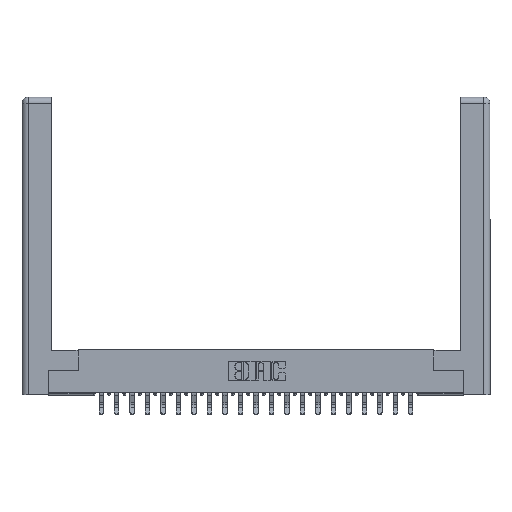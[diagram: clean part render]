
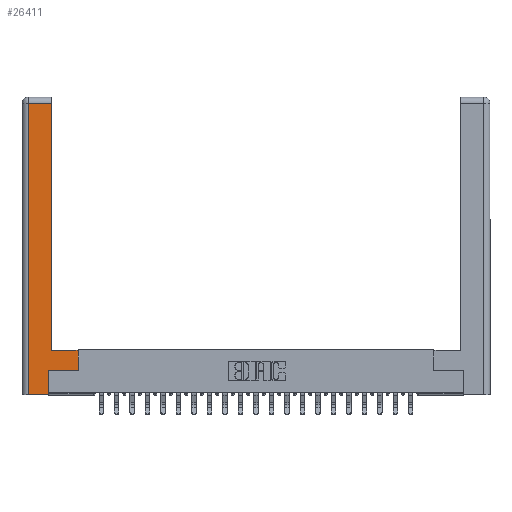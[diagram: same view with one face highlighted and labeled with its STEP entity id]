
A CAD part, top view. The second image highlights one B-rep face of the part: STEP entity #26411.
In plain terms, the highlighted planar face has unit normal (0, 0, 1).
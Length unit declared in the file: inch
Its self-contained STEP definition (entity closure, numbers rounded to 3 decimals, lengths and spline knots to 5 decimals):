
#15 = FACE_OUTER_BOUND ( 'NONE', #25318, .T. ) ;
#166 = ORIENTED_EDGE ( 'NONE', *, *, #12079, .T. ) ;
#227 = LINE ( 'NONE', #19545, #10065 ) ;
#1132 = CARTESIAN_POINT ( 'NONE',  ( 0.295, 0.45, 0. ) ) ;
#1381 = DIRECTION ( 'NONE',  ( 0., 1., 0. ) ) ;
#2128 = VERTEX_POINT ( 'NONE', #5772 ) ;
#2627 = ORIENTED_EDGE ( 'NONE', *, *, #8836, .T. ) ;
#3000 = EDGE_CURVE ( 'NONE', #23422, #21679, #227, .T. ) ;
#3068 = ORIENTED_EDGE ( 'NONE', *, *, #10850, .T. ) ;
#3162 = LINE ( 'NONE', #14942, #22546 ) ;
#4135 = EDGE_CURVE ( 'NONE', #21408, #21906, #3162, .T. ) ;
#4421 = DIRECTION ( 'NONE',  ( 0., -1., 0. ) ) ;
#4448 = ORIENTED_EDGE ( 'NONE', *, *, #3000, .T. ) ;
#5772 = CARTESIAN_POINT ( 'NONE',  ( 0.0615, 0., 0. ) ) ;
#6633 = DIRECTION ( 'NONE',  ( 0., 1., 0. ) ) ;
#8256 = CARTESIAN_POINT ( 'NONE',  ( 0.265, 0., 0. ) ) ;
#8334 = CARTESIAN_POINT ( 'NONE',  ( 0.565, 0.45, 0. ) ) ;
#8669 = DIRECTION ( 'NONE',  ( -1., 0., 0. ) ) ;
#8836 = EDGE_CURVE ( 'NONE', #23584, #11127, #10323, .T. ) ;
#9778 = VECTOR ( 'NONE', #18567, 39.37008 ) ;
#9855 = LINE ( 'NONE', #19994, #24811 ) ;
#10065 = VECTOR ( 'NONE', #6633, 39.37008 ) ;
#10323 = LINE ( 'NONE', #8334, #24931 ) ;
#10427 = DIRECTION ( 'NONE',  ( 0., 1., 0. ) ) ;
#10609 = DIRECTION ( 'NONE',  ( -1., 0., 0. ) ) ;
#10817 = AXIS2_PLACEMENT_3D ( 'NONE', #15261, #27907, #10609 ) ;
#10850 = EDGE_CURVE ( 'NONE', #2128, #23422, #20749, .T. ) ;
#11127 = VERTEX_POINT ( 'NONE', #22295 ) ;
#11364 = ORIENTED_EDGE ( 'NONE', *, *, #24656, .T. ) ;
#11489 = CARTESIAN_POINT ( 'NONE',  ( 0.295, 0.45, 0. ) ) ;
#11492 = LINE ( 'NONE', #20175, #9778 ) ;
#11603 = EDGE_CURVE ( 'NONE', #21906, #2128, #9855, .T. ) ;
#12079 = EDGE_CURVE ( 'NONE', #25902, #21408, #12204, .T. ) ;
#12204 = LINE ( 'NONE', #27332, #14255 ) ;
#12479 = ORIENTED_EDGE ( 'NONE', *, *, #16808, .T. ) ;
#12902 = DIRECTION ( 'NONE',  ( 1., 0., 0. ) ) ;
#13479 = CARTESIAN_POINT ( 'NONE',  ( 0.265, 0.245, 0. ) ) ;
#14255 = VECTOR ( 'NONE', #1381, 39.37008 ) ;
#14942 = CARTESIAN_POINT ( 'NONE',  ( 0.0615, 2.94, 0. ) ) ;
#15261 = CARTESIAN_POINT ( 'NONE',  ( 0., 0., 0. ) ) ;
#16410 = CARTESIAN_POINT ( 'NONE',  ( 0.565, 0.245, 0. ) ) ;
#16808 = EDGE_CURVE ( 'NONE', #11127, #25902, #18678, .T. ) ;
#17421 = ORIENTED_EDGE ( 'NONE', *, *, #4135, .T. ) ;
#18435 = DIRECTION ( 'NONE',  ( -1., 0., 0. ) ) ;
#18567 = DIRECTION ( 'NONE',  ( 1., 0., 0. ) ) ;
#18678 = LINE ( 'NONE', #1132, #20711 ) ;
#18765 = ORIENTED_EDGE ( 'NONE', *, *, #11603, .T. ) ;
#19545 = CARTESIAN_POINT ( 'NONE',  ( 0.265, 0.245, 0. ) ) ;
#19994 = CARTESIAN_POINT ( 'NONE',  ( 0.0615, 0., 0. ) ) ;
#20094 = VECTOR ( 'NONE', #12902, 39.37008 ) ;
#20175 = CARTESIAN_POINT ( 'NONE',  ( 0.565, 0.245, 0. ) ) ;
#20711 = VECTOR ( 'NONE', #18435, 39.37008 ) ;
#20749 = LINE ( 'NONE', #8256, #20094 ) ;
#21408 = VERTEX_POINT ( 'NONE', #25345 ) ;
#21679 = VERTEX_POINT ( 'NONE', #13479 ) ;
#21906 = VERTEX_POINT ( 'NONE', #24766 ) ;
#22295 = CARTESIAN_POINT ( 'NONE',  ( 0.565, 0.45, 0. ) ) ;
#22419 = CARTESIAN_POINT ( 'NONE',  ( 0.265, 0., 0. ) ) ;
#22546 = VECTOR ( 'NONE', #8669, 39.37008 ) ;
#23422 = VERTEX_POINT ( 'NONE', #22419 ) ;
#23584 = VERTEX_POINT ( 'NONE', #16410 ) ;
#23634 = PLANE ( 'NONE',  #10817 ) ;
#24656 = EDGE_CURVE ( 'NONE', #21679, #23584, #11492, .T. ) ;
#24766 = CARTESIAN_POINT ( 'NONE',  ( 0.0615, 2.94, 0. ) ) ;
#24811 = VECTOR ( 'NONE', #4421, 39.37008 ) ;
#24931 = VECTOR ( 'NONE', #10427, 39.37008 ) ;
#25318 = EDGE_LOOP ( 'NONE', ( #166, #17421, #18765, #3068, #4448, #11364, #2627, #12479 ) ) ;
#25345 = CARTESIAN_POINT ( 'NONE',  ( 0.295, 2.94, 0. ) ) ;
#25902 = VERTEX_POINT ( 'NONE', #11489 ) ;
#26411 = ADVANCED_FACE ( 'NONE', ( #15 ), #23634, .F. ) ;
#27332 = CARTESIAN_POINT ( 'NONE',  ( 0.295, 3., 0. ) ) ;
#27907 = DIRECTION ( 'NONE',  ( 0., 0., -1. ) ) ;
